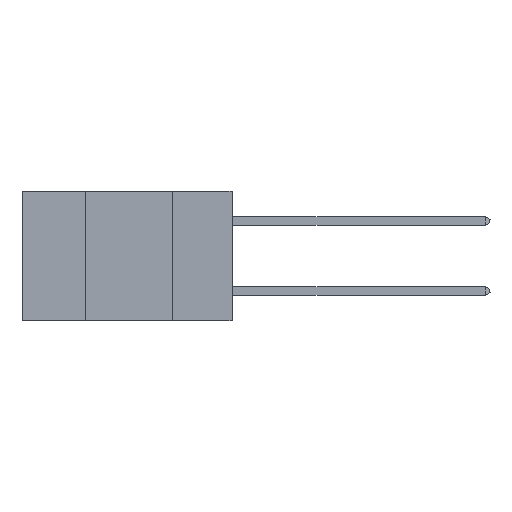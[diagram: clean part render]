
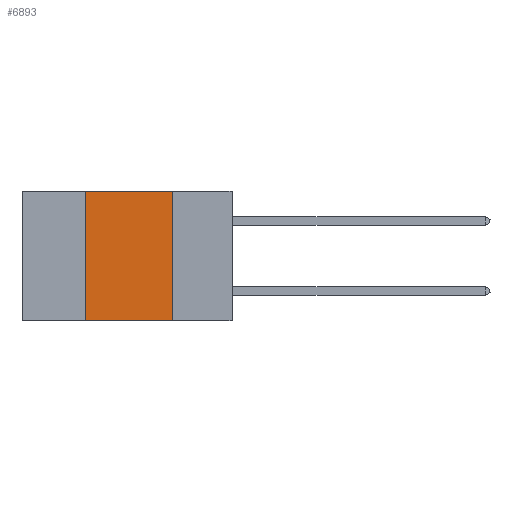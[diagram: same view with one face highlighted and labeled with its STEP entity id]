
A CAD part, left-side view. The second image highlights one B-rep face of the part: STEP entity #6893.
In plain terms, the highlighted planar face has unit normal (-1, 0, 0).
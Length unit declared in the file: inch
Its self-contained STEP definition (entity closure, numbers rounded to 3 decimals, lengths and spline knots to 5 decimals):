
#139 = ORIENTED_EDGE ( 'NONE', *, *, #34439, .T. ) ;
#1066 = FACE_OUTER_BOUND ( 'NONE', #21147, .T. ) ;
#4076 = DIRECTION ( 'NONE',  ( 0., 0., -1. ) ) ;
#4444 = EDGE_CURVE ( 'NONE', #35810, #32817, #43547, .T. ) ;
#6070 = DIRECTION ( 'NONE',  ( 0., -1., 0. ) ) ;
#6893 = ADVANCED_FACE ( 'NONE', ( #1066 ), #25898, .F. ) ;
#8710 = CARTESIAN_POINT ( 'NONE',  ( 0., 0.42, 0. ) ) ;
#11109 = CARTESIAN_POINT ( 'NONE',  ( 0., 0.17, -0.37 ) ) ;
#12160 = ORIENTED_EDGE ( 'NONE', *, *, #42235, .F. ) ;
#13675 = CARTESIAN_POINT ( 'NONE',  ( 0., 0.6, -0.37 ) ) ;
#13840 = DIRECTION ( 'NONE',  ( 0., -1., 0. ) ) ;
#13899 = CARTESIAN_POINT ( 'NONE',  ( 0., 0.42, 0. ) ) ;
#15073 = CARTESIAN_POINT ( 'NONE',  ( 0., 0.6, 0. ) ) ;
#15436 = ORIENTED_EDGE ( 'NONE', *, *, #4444, .F. ) ;
#20454 = CARTESIAN_POINT ( 'NONE',  ( 0., 0.17, 0. ) ) ;
#20671 = VERTEX_POINT ( 'NONE', #20454 ) ;
#20794 = CARTESIAN_POINT ( 'NONE',  ( 0., 0.6, 0. ) ) ;
#21147 = EDGE_LOOP ( 'NONE', ( #44888, #12160, #15436, #139 ) ) ;
#22602 = CARTESIAN_POINT ( 'NONE',  ( 0., 0.17, 0. ) ) ;
#25898 = PLANE ( 'NONE',  #29007 ) ;
#28897 = DIRECTION ( 'NONE',  ( 1., 0., 0. ) ) ;
#29007 = AXIS2_PLACEMENT_3D ( 'NONE', #15073, #28897, #4076 ) ;
#31975 = LINE ( 'NONE', #20794, #36494 ) ;
#32817 = VERTEX_POINT ( 'NONE', #13899 ) ;
#33960 = VECTOR ( 'NONE', #40615, 39.37008 ) ;
#34439 = EDGE_CURVE ( 'NONE', #35810, #45701, #40909, .T. ) ;
#35810 = VERTEX_POINT ( 'NONE', #44045 ) ;
#35811 = EDGE_CURVE ( 'NONE', #20671, #45701, #45000, .T. ) ;
#36494 = VECTOR ( 'NONE', #6070, 39.37008 ) ;
#36507 = VECTOR ( 'NONE', #43549, 39.37008 ) ;
#40317 = VECTOR ( 'NONE', #13840, 39.37008 ) ;
#40615 = DIRECTION ( 'NONE',  ( 0., 0., 1. ) ) ;
#40909 = LINE ( 'NONE', #13675, #40317 ) ;
#42235 = EDGE_CURVE ( 'NONE', #32817, #20671, #31975, .T. ) ;
#43547 = LINE ( 'NONE', #8710, #33960 ) ;
#43549 = DIRECTION ( 'NONE',  ( 0., 0., -1. ) ) ;
#44045 = CARTESIAN_POINT ( 'NONE',  ( 0., 0.42, -0.37 ) ) ;
#44888 = ORIENTED_EDGE ( 'NONE', *, *, #35811, .F. ) ;
#45000 = LINE ( 'NONE', #22602, #36507 ) ;
#45701 = VERTEX_POINT ( 'NONE', #11109 ) ;
